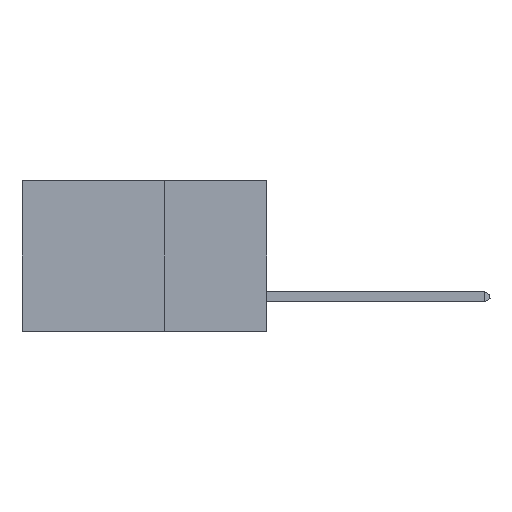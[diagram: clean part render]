
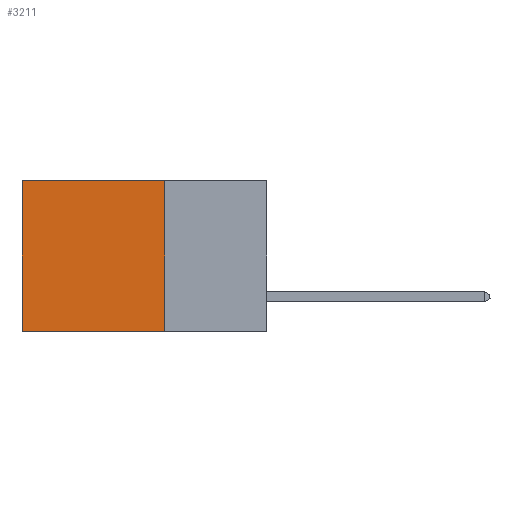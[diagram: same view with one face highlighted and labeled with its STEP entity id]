
A CAD part, left-side view. The second image highlights one B-rep face of the part: STEP entity #3211.
In plain terms, the highlighted planar face has unit normal (-1, 0, 0).
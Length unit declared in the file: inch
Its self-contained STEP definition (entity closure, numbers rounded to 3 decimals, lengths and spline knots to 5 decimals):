
#229 = CARTESIAN_POINT ( 'NONE',  ( 0.2875, 0.6, 0. ) ) ;
#947 = VECTOR ( 'NONE', #23404, 39.37008 ) ;
#1012 = EDGE_CURVE ( 'NONE', #6671, #18567, #21650, .T. ) ;
#1677 = ORIENTED_EDGE ( 'NONE', *, *, #1012, .T. ) ;
#1837 = DIRECTION ( 'NONE',  ( 0., 1., 0. ) ) ;
#1936 = ORIENTED_EDGE ( 'NONE', *, *, #18568, .F. ) ;
#2005 = CARTESIAN_POINT ( 'NONE',  ( 0.2875, 0.25, 0. ) ) ;
#3211 = ADVANCED_FACE ( 'NONE', ( #18699 ), #22705, .F. ) ;
#3389 = CARTESIAN_POINT ( 'NONE',  ( 0.2875, 0.25, 0. ) ) ;
#4287 = VERTEX_POINT ( 'NONE', #2005 ) ;
#4498 = DIRECTION ( 'NONE',  ( 0., 0., -1. ) ) ;
#5435 = CARTESIAN_POINT ( 'NONE',  ( 0.2875, 0.6, 0. ) ) ;
#5960 = CARTESIAN_POINT ( 'NONE',  ( 0.2875, 0.6, -0.37 ) ) ;
#6264 = LINE ( 'NONE', #3389, #21328 ) ;
#6671 = VERTEX_POINT ( 'NONE', #5435 ) ;
#6971 = VECTOR ( 'NONE', #1837, 39.37008 ) ;
#7987 = EDGE_LOOP ( 'NONE', ( #1677, #1936, #17101, #21709 ) ) ;
#8793 = EDGE_CURVE ( 'NONE', #4287, #6671, #6264, .T. ) ;
#8838 = DIRECTION ( 'NONE',  ( 1., 0., 0. ) ) ;
#10844 = DIRECTION ( 'NONE',  ( 0., 0., -1. ) ) ;
#11860 = CARTESIAN_POINT ( 'NONE',  ( 0.2875, 0.25, -0.37 ) ) ;
#15712 = VECTOR ( 'NONE', #4498, 39.37008 ) ;
#17056 = LINE ( 'NONE', #11860, #6971 ) ;
#17101 = ORIENTED_EDGE ( 'NONE', *, *, #19618, .F. ) ;
#17227 = CARTESIAN_POINT ( 'NONE',  ( 0.2875, 0.25, -0.37 ) ) ;
#18567 = VERTEX_POINT ( 'NONE', #5960 ) ;
#18568 = EDGE_CURVE ( 'NONE', #23728, #18567, #17056, .T. ) ;
#18699 = FACE_OUTER_BOUND ( 'NONE', #7987, .T. ) ;
#19188 = CARTESIAN_POINT ( 'NONE',  ( 0.2875, 0.25, 0. ) ) ;
#19618 = EDGE_CURVE ( 'NONE', #4287, #23728, #21075, .T. ) ;
#21075 = LINE ( 'NONE', #19188, #947 ) ;
#21328 = VECTOR ( 'NONE', #21451, 39.37008 ) ;
#21451 = DIRECTION ( 'NONE',  ( 0., 1., 0. ) ) ;
#21650 = LINE ( 'NONE', #229, #15712 ) ;
#21709 = ORIENTED_EDGE ( 'NONE', *, *, #8793, .T. ) ;
#22705 = PLANE ( 'NONE',  #23134 ) ;
#23134 = AXIS2_PLACEMENT_3D ( 'NONE', #24727, #8838, #10844 ) ;
#23404 = DIRECTION ( 'NONE',  ( 0., 0., -1. ) ) ;
#23728 = VERTEX_POINT ( 'NONE', #17227 ) ;
#24727 = CARTESIAN_POINT ( 'NONE',  ( 0.2875, 0.25, 0. ) ) ;
